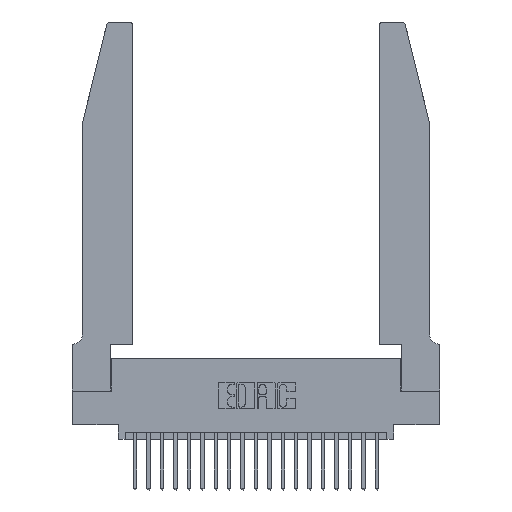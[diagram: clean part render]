
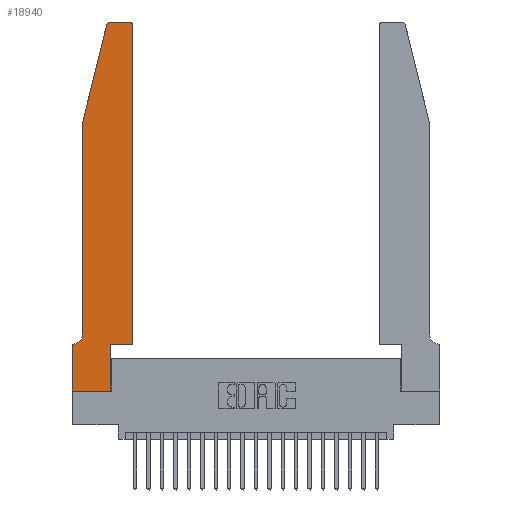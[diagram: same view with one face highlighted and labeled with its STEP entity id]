
A CAD part, top view. The second image highlights one B-rep face of the part: STEP entity #18940.
In plain terms, the highlighted planar face has unit normal (0, 0, 1).
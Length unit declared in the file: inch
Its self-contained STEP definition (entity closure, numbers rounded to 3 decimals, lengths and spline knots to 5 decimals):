
#24 = VERTEX_POINT ( 'NONE', #18382 ) ;
#71 = CARTESIAN_POINT ( 'NONE',  ( 0.2865, 0., 0.37 ) ) ;
#171 = CARTESIAN_POINT ( 'NONE',  ( 0.284, 2.75, 0.37 ) ) ;
#500 = ORIENTED_EDGE ( 'NONE', *, *, #13485, .T. ) ;
#598 = EDGE_CURVE ( 'NONE', #16811, #18391, #13413, .T. ) ;
#674 = LINE ( 'NONE', #8925, #18488 ) ;
#720 = ORIENTED_EDGE ( 'NONE', *, *, #21460, .T. ) ;
#833 = CARTESIAN_POINT ( 'NONE',  ( 0.0755, 2., 0.37 ) ) ;
#940 = CARTESIAN_POINT ( 'NONE',  ( 0., 0., 0.37 ) ) ;
#956 = PLANE ( 'NONE',  #11043 ) ;
#1191 = ORIENTED_EDGE ( 'NONE', *, *, #598, .T. ) ;
#1358 = DIRECTION ( 'NONE',  ( 0., 0., -1. ) ) ;
#1669 = EDGE_CURVE ( 'NONE', #5858, #9022, #2150, .T. ) ;
#1747 = CARTESIAN_POINT ( 'NONE',  ( 0.0755, 2., 0.37 ) ) ;
#1888 = CARTESIAN_POINT ( 'NONE',  ( 0.0755, 0.42, 0.37 ) ) ;
#2150 = CIRCLE ( 'NONE', #8288, 0.07 ) ;
#2474 = EDGE_CURVE ( 'NONE', #6508, #10623, #10058, .T. ) ;
#3052 = EDGE_CURVE ( 'NONE', #15039, #17932, #18222, .T. ) ;
#3177 = VERTEX_POINT ( 'NONE', #16216 ) ;
#3427 = CARTESIAN_POINT ( 'NONE',  ( 0.2865, 0.35, 0.37 ) ) ;
#3475 = DIRECTION ( 'NONE',  ( 1., 0., 0. ) ) ;
#3605 = ORIENTED_EDGE ( 'NONE', *, *, #6416, .T. ) ;
#3676 = ORIENTED_EDGE ( 'NONE', *, *, #1669, .T. ) ;
#4091 = EDGE_CURVE ( 'NONE', #24, #16811, #15748, .T. ) ;
#4147 = VECTOR ( 'NONE', #14062, 39.37008 ) ;
#4232 = VECTOR ( 'NONE', #16747, 39.37008 ) ;
#4368 = CARTESIAN_POINT ( 'NONE',  ( 0.4505, 0.35, 0.37 ) ) ;
#4664 = DIRECTION ( 'NONE',  ( 1., 0., 0. ) ) ;
#4961 = CARTESIAN_POINT ( 'NONE',  ( 0.4505, 0.35, 0.37 ) ) ;
#5264 = CARTESIAN_POINT ( 'NONE',  ( 0.284, 2.72, 0.37 ) ) ;
#5858 = VERTEX_POINT ( 'NONE', #1888 ) ;
#5901 = VECTOR ( 'NONE', #17869, 39.37008 ) ;
#5943 = VERTEX_POINT ( 'NONE', #171 ) ;
#6377 = AXIS2_PLACEMENT_3D ( 'NONE', #5264, #17558, #7075 ) ;
#6398 = VECTOR ( 'NONE', #15169, 39.37008 ) ;
#6416 = EDGE_CURVE ( 'NONE', #5943, #3177, #9610, .T. ) ;
#6499 = VECTOR ( 'NONE', #7140, 39.37008 ) ;
#6508 = VERTEX_POINT ( 'NONE', #17783 ) ;
#6723 = CARTESIAN_POINT ( 'NONE',  ( 0., 0., 0.37 ) ) ;
#7075 = DIRECTION ( 'NONE',  ( 1., 0., 0. ) ) ;
#7140 = DIRECTION ( 'NONE',  ( -1., 0., 0. ) ) ;
#7726 = CARTESIAN_POINT ( 'NONE',  ( 0.0755, 2., 0.37 ) ) ;
#8288 = AXIS2_PLACEMENT_3D ( 'NONE', #12140, #1358, #13888 ) ;
#8364 = CARTESIAN_POINT ( 'NONE',  ( 0.4205, 2.75, 0.37 ) ) ;
#8668 = VECTOR ( 'NONE', #18956, 39.37008 ) ;
#8925 = CARTESIAN_POINT ( 'NONE',  ( 0.2605, 2.75, 0.37 ) ) ;
#9022 = VERTEX_POINT ( 'NONE', #19959 ) ;
#9610 = CIRCLE ( 'NONE', #6377, 0.03 ) ;
#10058 = LINE ( 'NONE', #16161, #5901 ) ;
#10623 = VERTEX_POINT ( 'NONE', #940 ) ;
#11043 = AXIS2_PLACEMENT_3D ( 'NONE', #15214, #15285, #4664 ) ;
#11626 = VECTOR ( 'NONE', #17289, 39.37008 ) ;
#11927 = AXIS2_PLACEMENT_3D ( 'NONE', #22104, #19927, #3475 ) ;
#12140 = CARTESIAN_POINT ( 'NONE',  ( 0.0055, 0.42, 0.37 ) ) ;
#12396 = CARTESIAN_POINT ( 'NONE',  ( 0.0755, 0.35, 0.37 ) ) ;
#12476 = ORIENTED_EDGE ( 'NONE', *, *, #19180, .T. ) ;
#13316 = LINE ( 'NONE', #6723, #8668 ) ;
#13386 = ORIENTED_EDGE ( 'NONE', *, *, #13814, .T. ) ;
#13413 = CIRCLE ( 'NONE', #11927, 0.03 ) ;
#13485 = EDGE_CURVE ( 'NONE', #17932, #24, #17759, .T. ) ;
#13778 = ORIENTED_EDGE ( 'NONE', *, *, #20816, .T. ) ;
#13814 = EDGE_CURVE ( 'NONE', #9022, #6508, #20440, .T. ) ;
#13888 = DIRECTION ( 'NONE',  ( -1., 0., 0. ) ) ;
#14062 = DIRECTION ( 'NONE',  ( 0., 1., 0. ) ) ;
#15039 = VERTEX_POINT ( 'NONE', #71 ) ;
#15152 = VERTEX_POINT ( 'NONE', #7726 ) ;
#15169 = DIRECTION ( 'NONE',  ( 0., -1., 0. ) ) ;
#15214 = CARTESIAN_POINT ( 'NONE',  ( 0., 0.35, 0.37 ) ) ;
#15285 = DIRECTION ( 'NONE',  ( 0., 0., 1. ) ) ;
#15748 = LINE ( 'NONE', #4961, #11626 ) ;
#15838 = CARTESIAN_POINT ( 'NONE',  ( 0.2865, 0.35, 0.37 ) ) ;
#15897 = DIRECTION ( 'NONE',  ( -1., 0., 0. ) ) ;
#15956 = ORIENTED_EDGE ( 'NONE', *, *, #3052, .T. ) ;
#16030 = EDGE_CURVE ( 'NONE', #10623, #15039, #13316, .T. ) ;
#16037 = DIRECTION ( 'NONE',  ( -0.239, -0.971, 0. ) ) ;
#16161 = CARTESIAN_POINT ( 'NONE',  ( 0., 0., 0.37 ) ) ;
#16216 = CARTESIAN_POINT ( 'NONE',  ( 0.25487, 2.72718, 0.37 ) ) ;
#16377 = CARTESIAN_POINT ( 'NONE',  ( 0.4505, 2.72, 0.37 ) ) ;
#16747 = DIRECTION ( 'NONE',  ( 1., 0., 0. ) ) ;
#16811 = VERTEX_POINT ( 'NONE', #16377 ) ;
#17289 = DIRECTION ( 'NONE',  ( 0., 1., 0. ) ) ;
#17441 = ORIENTED_EDGE ( 'NONE', *, *, #2474, .T. ) ;
#17558 = DIRECTION ( 'NONE',  ( 0., 0., 1. ) ) ;
#17741 = ORIENTED_EDGE ( 'NONE', *, *, #16030, .T. ) ;
#17759 = LINE ( 'NONE', #4368, #4232 ) ;
#17783 = CARTESIAN_POINT ( 'NONE',  ( 0., 0.35, 0.37 ) ) ;
#17869 = DIRECTION ( 'NONE',  ( 0., -1., 0. ) ) ;
#17932 = VERTEX_POINT ( 'NONE', #3427 ) ;
#18222 = LINE ( 'NONE', #15838, #4147 ) ;
#18295 = VECTOR ( 'NONE', #16037, 39.37008 ) ;
#18382 = CARTESIAN_POINT ( 'NONE',  ( 0.4505, 0.35, 0.37 ) ) ;
#18391 = VERTEX_POINT ( 'NONE', #8364 ) ;
#18488 = VECTOR ( 'NONE', #15897, 39.37008 ) ;
#18940 = ADVANCED_FACE ( 'NONE', ( #22836 ), #956, .T. ) ;
#18956 = DIRECTION ( 'NONE',  ( 1., 0., 0. ) ) ;
#19180 = EDGE_CURVE ( 'NONE', #3177, #15152, #19604, .T. ) ;
#19462 = ORIENTED_EDGE ( 'NONE', *, *, #4091, .T. ) ;
#19604 = LINE ( 'NONE', #1747, #18295 ) ;
#19927 = DIRECTION ( 'NONE',  ( 0., 0., 1. ) ) ;
#19959 = CARTESIAN_POINT ( 'NONE',  ( 0.0055, 0.35, 0.37 ) ) ;
#20222 = EDGE_LOOP ( 'NONE', ( #13778, #3605, #12476, #720, #3676, #13386, #17441, #17741, #15956, #500, #19462, #1191 ) ) ;
#20440 = LINE ( 'NONE', #12396, #6499 ) ;
#20816 = EDGE_CURVE ( 'NONE', #18391, #5943, #674, .T. ) ;
#20893 = LINE ( 'NONE', #833, #6398 ) ;
#21460 = EDGE_CURVE ( 'NONE', #15152, #5858, #20893, .T. ) ;
#22104 = CARTESIAN_POINT ( 'NONE',  ( 0.4205, 2.72, 0.37 ) ) ;
#22836 = FACE_OUTER_BOUND ( 'NONE', #20222, .T. ) ;
